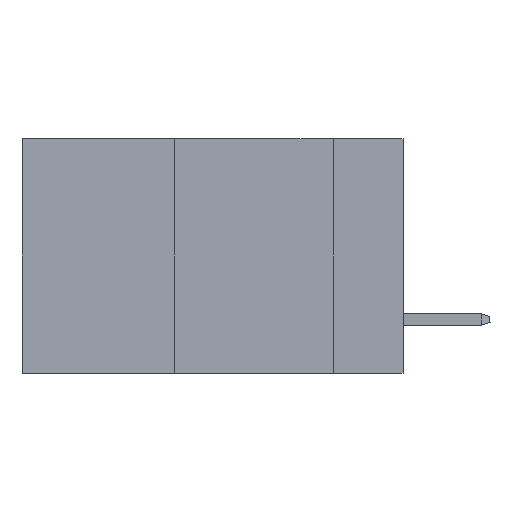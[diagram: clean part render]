
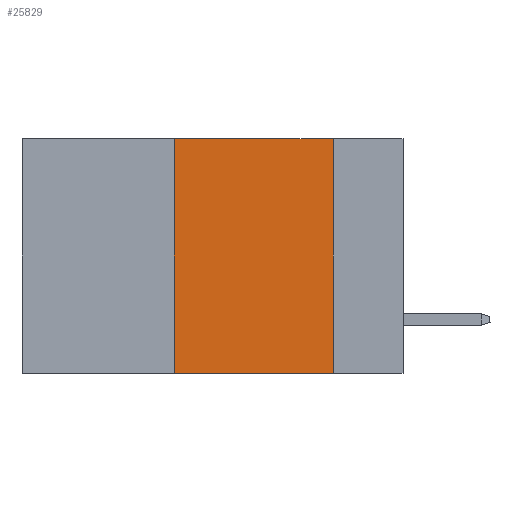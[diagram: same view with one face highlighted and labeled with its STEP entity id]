
A CAD part, left-side view. The second image highlights one B-rep face of the part: STEP entity #25829.
In plain terms, the highlighted planar face has unit normal (-1, 0, 0).
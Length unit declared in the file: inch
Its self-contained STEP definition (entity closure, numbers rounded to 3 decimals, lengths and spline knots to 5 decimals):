
#172 = LINE ( 'NONE', #12274, #7821 ) ;
#530 = CARTESIAN_POINT ( 'NONE',  ( 0., 0.36, 0. ) ) ;
#639 = VERTEX_POINT ( 'NONE', #14326 ) ;
#793 = DIRECTION ( 'NONE',  ( 0., -1., 0. ) ) ;
#1077 = DIRECTION ( 'NONE',  ( 1., 0., 0. ) ) ;
#1578 = ORIENTED_EDGE ( 'NONE', *, *, #16001, .T. ) ;
#1939 = VECTOR ( 'NONE', #34323, 39.37008 ) ;
#3136 = EDGE_CURVE ( 'NONE', #31727, #9744, #31181, .T. ) ;
#4600 = VERTEX_POINT ( 'NONE', #33571 ) ;
#6556 = LINE ( 'NONE', #28258, #1939 ) ;
#7821 = VECTOR ( 'NONE', #24343, 39.37008 ) ;
#7906 = FACE_OUTER_BOUND ( 'NONE', #9841, .T. ) ;
#8443 = ORIENTED_EDGE ( 'NONE', *, *, #9585, .F. ) ;
#9338 = DIRECTION ( 'NONE',  ( 0., 0., -1. ) ) ;
#9585 = EDGE_CURVE ( 'NONE', #4600, #31727, #172, .T. ) ;
#9744 = VERTEX_POINT ( 'NONE', #26448 ) ;
#9841 = EDGE_LOOP ( 'NONE', ( #9901, #18368, #8443, #1578 ) ) ;
#9901 = ORIENTED_EDGE ( 'NONE', *, *, #12870, .F. ) ;
#10610 = VECTOR ( 'NONE', #9338, 39.37008 ) ;
#12274 = CARTESIAN_POINT ( 'NONE',  ( 0., 0.36, 0. ) ) ;
#12870 = EDGE_CURVE ( 'NONE', #9744, #639, #28413, .T. ) ;
#14326 = CARTESIAN_POINT ( 'NONE',  ( 0., 0.11, -0.37 ) ) ;
#16001 = EDGE_CURVE ( 'NONE', #4600, #639, #6556, .T. ) ;
#16169 = CARTESIAN_POINT ( 'NONE',  ( 0., 0.6, 0. ) ) ;
#18368 = ORIENTED_EDGE ( 'NONE', *, *, #3136, .F. ) ;
#20175 = PLANE ( 'NONE',  #29686 ) ;
#24343 = DIRECTION ( 'NONE',  ( 0., 0., 1. ) ) ;
#25829 = ADVANCED_FACE ( 'NONE', ( #7906 ), #20175, .F. ) ;
#26448 = CARTESIAN_POINT ( 'NONE',  ( 0., 0.11, 0. ) ) ;
#28258 = CARTESIAN_POINT ( 'NONE',  ( 0., 0.6, -0.37 ) ) ;
#28413 = LINE ( 'NONE', #34275, #10610 ) ;
#28416 = DIRECTION ( 'NONE',  ( 0., 0., -1. ) ) ;
#29686 = AXIS2_PLACEMENT_3D ( 'NONE', #16169, #1077, #28416 ) ;
#31181 = LINE ( 'NONE', #37443, #32475 ) ;
#31727 = VERTEX_POINT ( 'NONE', #530 ) ;
#32475 = VECTOR ( 'NONE', #793, 39.37008 ) ;
#33571 = CARTESIAN_POINT ( 'NONE',  ( 0., 0.36, -0.37 ) ) ;
#34275 = CARTESIAN_POINT ( 'NONE',  ( 0., 0.11, 0. ) ) ;
#34323 = DIRECTION ( 'NONE',  ( 0., -1., 0. ) ) ;
#37443 = CARTESIAN_POINT ( 'NONE',  ( 0., 0.6, 0. ) ) ;
